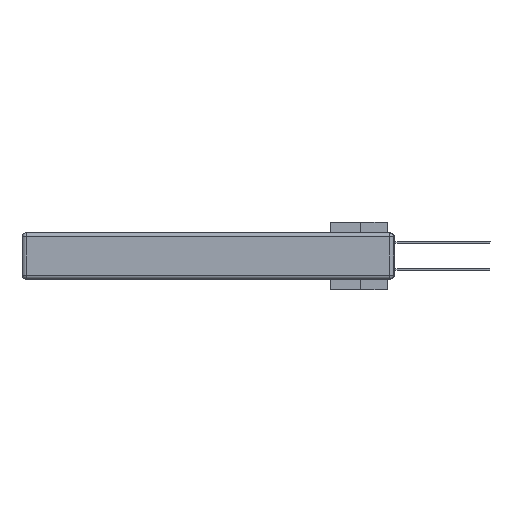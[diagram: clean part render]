
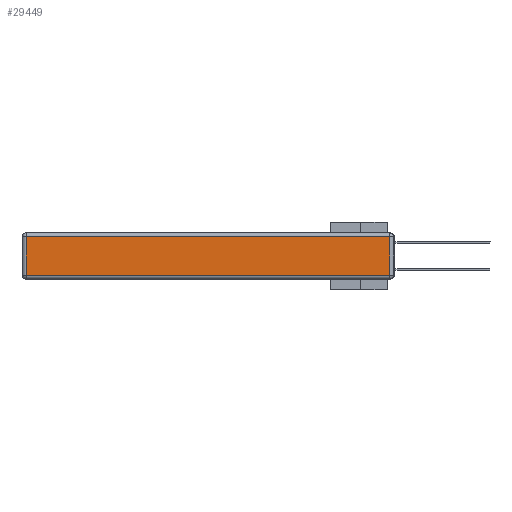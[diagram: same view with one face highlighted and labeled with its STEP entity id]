
A CAD part, left-side view. The second image highlights one B-rep face of the part: STEP entity #29449.
In plain terms, the highlighted planar face has unit normal (-1, 0, 0).
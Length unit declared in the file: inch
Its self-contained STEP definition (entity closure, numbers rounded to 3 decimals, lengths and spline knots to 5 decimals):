
#181 = VECTOR ( 'NONE', #2527, 39.37008 ) ;
#415 = ORIENTED_EDGE ( 'NONE', *, *, #13036, .T. ) ;
#1721 = CARTESIAN_POINT ( 'NONE',  ( 0., 0., -0.343 ) ) ;
#2527 = DIRECTION ( 'NONE',  ( 0., 0., -1. ) ) ;
#3632 = LINE ( 'NONE', #17423, #8054 ) ;
#4305 = ORIENTED_EDGE ( 'NONE', *, *, #8058, .T. ) ;
#5071 = ORIENTED_EDGE ( 'NONE', *, *, #8351, .T. ) ;
#6780 = CARTESIAN_POINT ( 'NONE',  ( 0., 2.75, -0.03 ) ) ;
#6861 = EDGE_CURVE ( 'NONE', #29694, #20516, #3632, .T. ) ;
#7506 = CARTESIAN_POINT ( 'NONE',  ( 0., 0.03, -0.343 ) ) ;
#8054 = VECTOR ( 'NONE', #28611, 39.37008 ) ;
#8058 = EDGE_CURVE ( 'NONE', #20255, #29834, #18153, .T. ) ;
#8351 = EDGE_CURVE ( 'NONE', #29834, #29694, #28039, .T. ) ;
#9807 = FACE_OUTER_BOUND ( 'NONE', #25419, .T. ) ;
#10262 = VECTOR ( 'NONE', #30443, 39.37008 ) ;
#13036 = EDGE_CURVE ( 'NONE', #20516, #20255, #24763, .T. ) ;
#15142 = PLANE ( 'NONE',  #24869 ) ;
#15859 = DIRECTION ( 'NONE',  ( 0., 0., 1. ) ) ;
#17423 = CARTESIAN_POINT ( 'NONE',  ( 0., 0., -0.313 ) ) ;
#18153 = LINE ( 'NONE', #6780, #28886 ) ;
#19519 = CARTESIAN_POINT ( 'NONE',  ( 0., 2.72, -0.313 ) ) ;
#20255 = VERTEX_POINT ( 'NONE', #22049 ) ;
#20516 = VERTEX_POINT ( 'NONE', #34317 ) ;
#22049 = CARTESIAN_POINT ( 'NONE',  ( 0., 0.03, -0.03 ) ) ;
#22197 = CARTESIAN_POINT ( 'NONE',  ( 0., 2.72, -0.03 ) ) ;
#24183 = ORIENTED_EDGE ( 'NONE', *, *, #6861, .T. ) ;
#24763 = LINE ( 'NONE', #7506, #10262 ) ;
#24869 = AXIS2_PLACEMENT_3D ( 'NONE', #1721, #34770, #15859 ) ;
#25419 = EDGE_LOOP ( 'NONE', ( #24183, #415, #4305, #5071 ) ) ;
#26434 = DIRECTION ( 'NONE',  ( 0., 1., 0. ) ) ;
#28039 = LINE ( 'NONE', #28219, #181 ) ;
#28219 = CARTESIAN_POINT ( 'NONE',  ( 0., 2.72, -0.343 ) ) ;
#28611 = DIRECTION ( 'NONE',  ( 0., -1., 0. ) ) ;
#28886 = VECTOR ( 'NONE', #26434, 39.37008 ) ;
#29449 = ADVANCED_FACE ( 'NONE', ( #9807 ), #15142, .T. ) ;
#29694 = VERTEX_POINT ( 'NONE', #19519 ) ;
#29834 = VERTEX_POINT ( 'NONE', #22197 ) ;
#30443 = DIRECTION ( 'NONE',  ( 0., 0., 1. ) ) ;
#34317 = CARTESIAN_POINT ( 'NONE',  ( 0., 0.03, -0.313 ) ) ;
#34770 = DIRECTION ( 'NONE',  ( -1., 0., 0. ) ) ;
